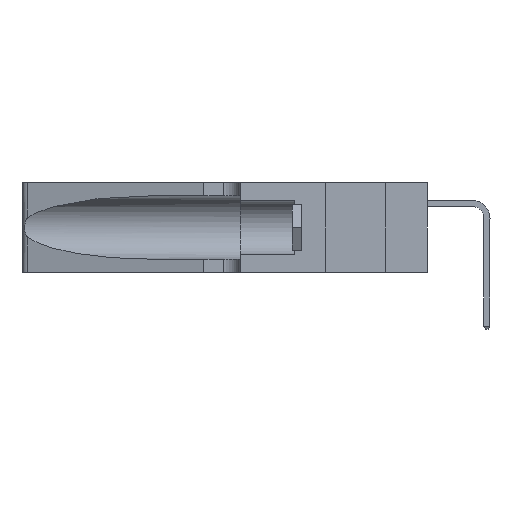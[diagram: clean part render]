
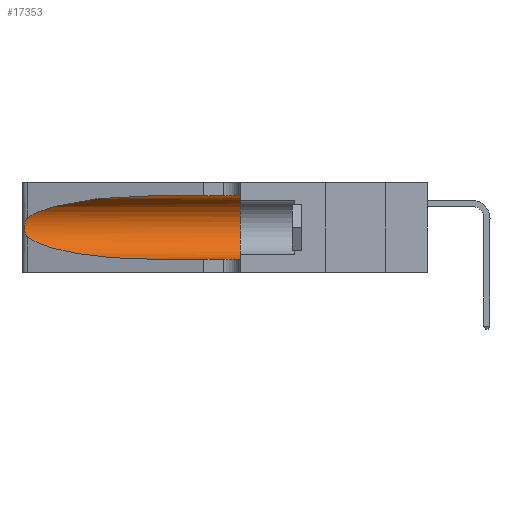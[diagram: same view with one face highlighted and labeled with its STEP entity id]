
A CAD part, left-side view. The second image highlights one B-rep face of the part: STEP entity #17353.
In plain terms, the highlighted cylindrical face has radius 3.308 mm (diameter 6.617 mm), a partial arc.
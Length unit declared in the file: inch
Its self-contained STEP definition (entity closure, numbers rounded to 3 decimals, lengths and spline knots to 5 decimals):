
#275 = VERTEX_POINT ( 'NONE', #21883 ) ;
#1061 = EDGE_CURVE ( 'NONE', #2499, #4854, #22067, .T. ) ;
#1172 = CARTESIAN_POINT ( 'NONE',  ( 0.26017, 1.23833, 0.17102 ) ) ;
#1542 = ORIENTED_EDGE ( 'NONE', *, *, #15068, .T. ) ;
#1618 = CARTESIAN_POINT ( 'NONE',  ( 0.25487, 1.22718, 0.22369 ) ) ;
#1775 = ORIENTED_EDGE ( 'NONE', *, *, #20882, .T. ) ;
#2105 = CIRCLE ( 'NONE', #16127, 0.13025 ) ;
#2499 = VERTEX_POINT ( 'NONE', #14712 ) ;
#2921 = CARTESIAN_POINT ( 'NONE',  ( 0.25789, 1.23486, 0.15765 ) ) ;
#4198 = CARTESIAN_POINT ( 'NONE',  ( 0.25487, 1.22718, 0.14631 ) ) ;
#4389 = ORIENTED_EDGE ( 'NONE', *, *, #12761, .T. ) ;
#4633 = CARTESIAN_POINT ( 'NONE',  ( 0.25555, 1.22993, 0.14849 ) ) ;
#4854 = VERTEX_POINT ( 'NONE', #21917 ) ;
#5382 = CARTESIAN_POINT ( 'NONE',  ( 0.1305, 0.35, 0.185 ) ) ;
#5383 = ORIENTED_EDGE ( 'NONE', *, *, #16917, .F. ) ;
#6157 = CYLINDRICAL_SURFACE ( 'NONE', #8412, 0.13025 ) ;
#6526 = CARTESIAN_POINT ( 'NONE',  ( 0.1305, 1.61858, 0.185 ) ) ;
#7172 = DIRECTION ( 'NONE',  ( 0., 0., 1. ) ) ;
#7277 = FACE_OUTER_BOUND ( 'NONE', #16391, .T. ) ;
#7745 = VECTOR ( 'NONE', #22199, 39.37008 ) ;
#7758 = CARTESIAN_POINT ( 'NONE',  ( 0.1305, 0.72297, 0.05475 ) ) ;
#7964 = CARTESIAN_POINT ( 'NONE',  ( 0.1305, 0.72297, 0.31525 ) ) ;
#8123 = CARTESIAN_POINT ( 'NONE',  ( 0.25787, 1.23484, 0.2124 ) ) ;
#8412 = AXIS2_PLACEMENT_3D ( 'NONE', #6526, #20170, #21791 ) ;
#8603 = CARTESIAN_POINT ( 'NONE',  ( 0.1305, 1.61858, 0.31525 ) ) ;
#8892 = CARTESIAN_POINT ( 'NONE',  ( 0.1305, 1.61858, 0.05475 ) ) ;
#9315 = VERTEX_POINT ( 'NONE', #9515 ) ;
#9515 = CARTESIAN_POINT ( 'NONE',  ( 0.1305, 0.72297, 0.31525 ) ) ;
#9593 = VECTOR ( 'NONE', #11465, 39.37008 ) ;
#9702 = CARTESIAN_POINT ( 'NONE',  ( 0.18966, 0.96281, 0.31525 ) ) ;
#9703 = ORIENTED_EDGE ( 'NONE', *, *, #18596, .F. ) ;
#9784 = CARTESIAN_POINT ( 'NONE',  ( 0.25487, 1.22718, 0.22369 ) ) ;
#9862 = CARTESIAN_POINT ( 'NONE',  ( 0.26018, 1.23835, 0.19895 ) ) ;
#11465 = DIRECTION ( 'NONE',  ( 0., -1., 0. ) ) ;
#11596 = CARTESIAN_POINT ( 'NONE',  ( 0.26075, 1.23896, 0.178 ) ) ;
#12339 = LINE ( 'NONE', #8603, #7745 ) ;
#12761 = EDGE_CURVE ( 'NONE', #21877, #2499, #19479, .T. ) ;
#13297 = CARTESIAN_POINT ( 'NONE',  ( 0.25856, 1.23593, 0.16098 ) ) ;
#14584 = CARTESIAN_POINT ( 'NONE',  ( 0.2373, 1.15595, 0.08982 ) ) ;
#14712 = CARTESIAN_POINT ( 'NONE',  ( 0.1305, 0.72297, 0.05475 ) ) ;
#14915 = CARTESIAN_POINT ( 'NONE',  ( 0.25487, 1.22718, 0.22369 ) ) ;
#14989 = CARTESIAN_POINT ( 'NONE',  ( 0.25639, 1.23186, 0.15144 ) ) ;
#15068 = EDGE_CURVE ( 'NONE', #9315, #18064, #15918, .T. ) ;
#15918 =( BOUNDED_CURVE ( )  B_SPLINE_CURVE ( 3, ( #7964, #9702, #19933, #9784 ),
 .UNSPECIFIED., .F., .F. ) 
 B_SPLINE_CURVE_WITH_KNOTS ( ( 4, 4 ),
 ( 1.5708, 2.84003 ),
 .UNSPECIFIED. ) 
 CURVE ( )  GEOMETRIC_REPRESENTATION_ITEM ( )  RATIONAL_B_SPLINE_CURVE ( ( 1., 0.87, 0.87, 1. ) ) 
 REPRESENTATION_ITEM ( '' )  );
#16127 = AXIS2_PLACEMENT_3D ( 'NONE', #5382, #17403, #7172 ) ;
#16391 = EDGE_LOOP ( 'NONE', ( #1542, #1775, #4389, #20571, #5383, #9703 ) ) ;
#16571 = CARTESIAN_POINT ( 'NONE',  ( 0.25487, 1.22718, 0.14631 ) ) ;
#16700 = CARTESIAN_POINT ( 'NONE',  ( 0.25487, 1.22718, 0.14631 ) ) ;
#16917 = EDGE_CURVE ( 'NONE', #275, #4854, #2105, .T. ) ;
#17353 = ADVANCED_FACE ( 'NONE', ( #7277 ), #6157, .F. ) ;
#17403 = DIRECTION ( 'NONE',  ( 0., 1., 0. ) ) ;
#17975 = CARTESIAN_POINT ( 'NONE',  ( 0.18966, 0.96281, 0.05475 ) ) ;
#18064 = VERTEX_POINT ( 'NONE', #1618 ) ;
#18178 = CARTESIAN_POINT ( 'NONE',  ( 0.25555, 1.22994, 0.2215 ) ) ;
#18321 = CARTESIAN_POINT ( 'NONE',  ( 0.25639, 1.23184, 0.21858 ) ) ;
#18596 = EDGE_CURVE ( 'NONE', #9315, #275, #12339, .T. ) ;
#19479 =( BOUNDED_CURVE ( )  B_SPLINE_CURVE ( 3, ( #4198, #14584, #17975, #7758 ),
 .UNSPECIFIED., .F., .T. ) 
 B_SPLINE_CURVE_WITH_KNOTS ( ( 4, 4 ),
 ( 3.44316, 4.71239 ),
 .UNSPECIFIED. ) 
 CURVE ( )  GEOMETRIC_REPRESENTATION_ITEM ( )  RATIONAL_B_SPLINE_CURVE ( ( 1., 0.87, 0.87, 1. ) ) 
 REPRESENTATION_ITEM ( '' )  );
#19933 = CARTESIAN_POINT ( 'NONE',  ( 0.2373, 1.15595, 0.28018 ) ) ;
#20007 = CARTESIAN_POINT ( 'NONE',  ( 0.25854, 1.2359, 0.20912 ) ) ;
#20170 = DIRECTION ( 'NONE',  ( 0., -1., 0. ) ) ;
#20571 = ORIENTED_EDGE ( 'NONE', *, *, #1061, .T. ) ;
#20882 = EDGE_CURVE ( 'NONE', #18064, #21877, #22140, .T. ) ;
#21709 = CARTESIAN_POINT ( 'NONE',  ( 0.26075, 1.23896, 0.19203 ) ) ;
#21791 = DIRECTION ( 'NONE',  ( 0., 0., -1. ) ) ;
#21877 = VERTEX_POINT ( 'NONE', #16571 ) ;
#21883 = CARTESIAN_POINT ( 'NONE',  ( 0.1305, 0.35, 0.31525 ) ) ;
#21917 = CARTESIAN_POINT ( 'NONE',  ( 0.1305, 0.35, 0.05475 ) ) ;
#22067 = LINE ( 'NONE', #8892, #9593 ) ;
#22140 = B_SPLINE_CURVE_WITH_KNOTS ( 'NONE', 3,
 ( #14915, #18178, #18321, #8123, #20007, #9862, #21709, #11596, #1172, #13297, #2921, #14989, #4633, #16700 ),
 .UNSPECIFIED., .F., .F.,
 ( 4, 2, 2, 2, 2, 2, 4 ),
 ( 0., 0.00027, 0.00053, 0.00107, 0.0016, 0.00187, 0.00214 ),
 .UNSPECIFIED. ) ;
#22199 = DIRECTION ( 'NONE',  ( 0., -1., 0. ) ) ;
